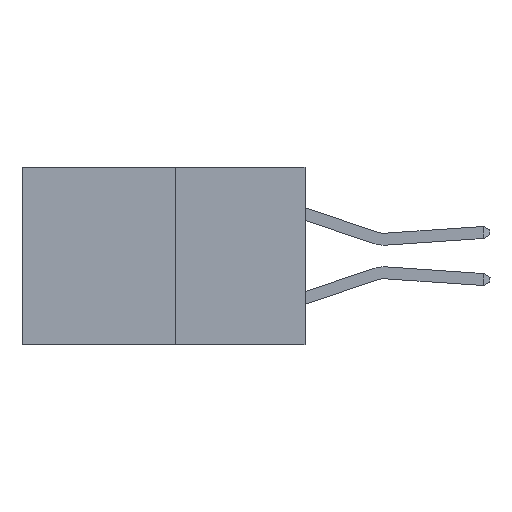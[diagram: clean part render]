
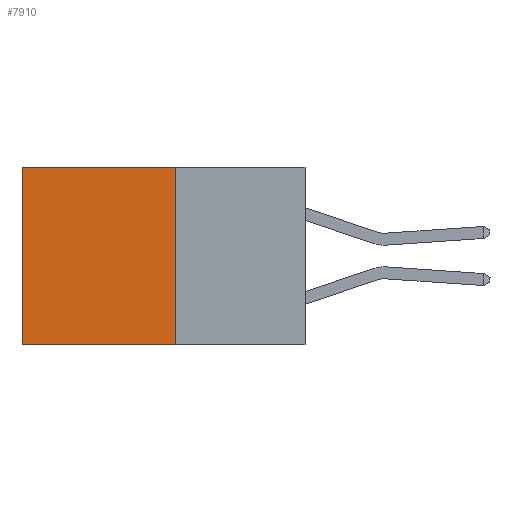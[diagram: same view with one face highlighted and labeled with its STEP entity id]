
A CAD part, left-side view. The second image highlights one B-rep face of the part: STEP entity #7910.
In plain terms, the highlighted planar face has unit normal (-1, 0, 0).
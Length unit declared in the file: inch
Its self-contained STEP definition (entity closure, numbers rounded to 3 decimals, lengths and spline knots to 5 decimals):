
#45 = CARTESIAN_POINT ( 'NONE',  ( 0.277, 0.27, -0.37 ) ) ;
#478 = VERTEX_POINT ( 'NONE', #45 ) ;
#1519 = ORIENTED_EDGE ( 'NONE', *, *, #12047, .T. ) ;
#2237 = FACE_OUTER_BOUND ( 'NONE', #9326, .T. ) ;
#2369 = CARTESIAN_POINT ( 'NONE',  ( 0.277, 0.59, 0. ) ) ;
#2646 = LINE ( 'NONE', #13085, #13185 ) ;
#3190 = CARTESIAN_POINT ( 'NONE',  ( 0.277, 0.27, 0. ) ) ;
#3491 = CARTESIAN_POINT ( 'NONE',  ( 0.277, 0.59, -0.37 ) ) ;
#3671 = DIRECTION ( 'NONE',  ( 0., 1., 0. ) ) ;
#4186 = AXIS2_PLACEMENT_3D ( 'NONE', #11828, #11878, #5781 ) ;
#4553 = DIRECTION ( 'NONE',  ( 0., 0., -1. ) ) ;
#4642 = VECTOR ( 'NONE', #7366, 39.37008 ) ;
#4720 = PLANE ( 'NONE',  #4186 ) ;
#5781 = DIRECTION ( 'NONE',  ( 0., 0., -1. ) ) ;
#6016 = DIRECTION ( 'NONE',  ( 0., 0., -1. ) ) ;
#6426 = ORIENTED_EDGE ( 'NONE', *, *, #11147, .T. ) ;
#7366 = DIRECTION ( 'NONE',  ( 0., 1., 0. ) ) ;
#7810 = VERTEX_POINT ( 'NONE', #12738 ) ;
#7910 = ADVANCED_FACE ( 'NONE', ( #2237 ), #4720, .F. ) ;
#7921 = LINE ( 'NONE', #3491, #9977 ) ;
#8308 = VERTEX_POINT ( 'NONE', #13187 ) ;
#9172 = ORIENTED_EDGE ( 'NONE', *, *, #12960, .F. ) ;
#9326 = EDGE_LOOP ( 'NONE', ( #6426, #9172, #9485, #1519 ) ) ;
#9485 = ORIENTED_EDGE ( 'NONE', *, *, #13105, .F. ) ;
#9977 = VECTOR ( 'NONE', #4553, 39.37008 ) ;
#10098 = LINE ( 'NONE', #11891, #12437 ) ;
#10121 = LINE ( 'NONE', #3190, #4642 ) ;
#11147 = EDGE_CURVE ( 'NONE', #11539, #7810, #7921, .T. ) ;
#11539 = VERTEX_POINT ( 'NONE', #2369 ) ;
#11828 = CARTESIAN_POINT ( 'NONE',  ( 0.277, 0.27, -0.37 ) ) ;
#11878 = DIRECTION ( 'NONE',  ( 1., 0., 0. ) ) ;
#11891 = CARTESIAN_POINT ( 'NONE',  ( 0.277, 0.27, -0.37 ) ) ;
#12047 = EDGE_CURVE ( 'NONE', #8308, #11539, #10121, .T. ) ;
#12437 = VECTOR ( 'NONE', #3671, 39.37008 ) ;
#12738 = CARTESIAN_POINT ( 'NONE',  ( 0.277, 0.59, -0.37 ) ) ;
#12960 = EDGE_CURVE ( 'NONE', #478, #7810, #10098, .T. ) ;
#13085 = CARTESIAN_POINT ( 'NONE',  ( 0.277, 0.27, -0.37 ) ) ;
#13105 = EDGE_CURVE ( 'NONE', #8308, #478, #2646, .T. ) ;
#13185 = VECTOR ( 'NONE', #6016, 39.37008 ) ;
#13187 = CARTESIAN_POINT ( 'NONE',  ( 0.277, 0.27, 0. ) ) ;
